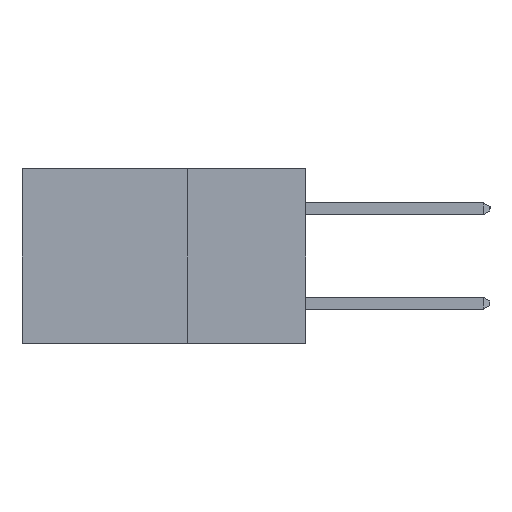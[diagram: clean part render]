
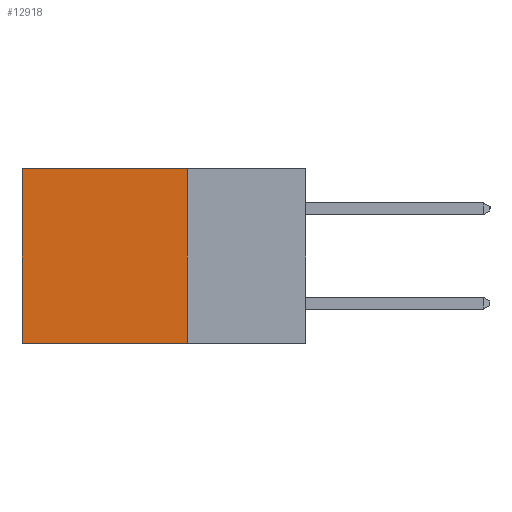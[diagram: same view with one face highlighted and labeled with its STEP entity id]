
A CAD part, left-side view. The second image highlights one B-rep face of the part: STEP entity #12918.
In plain terms, the highlighted planar face has unit normal (-1, 0, 0).
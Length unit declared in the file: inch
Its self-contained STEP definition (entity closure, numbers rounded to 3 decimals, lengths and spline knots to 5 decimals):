
#1525 = ORIENTED_EDGE ( 'NONE', *, *, #2690, .T. ) ;
#2541 = LINE ( 'NONE', #11720, #13018 ) ;
#2690 = EDGE_CURVE ( 'NONE', #2860, #10232, #7359, .T. ) ;
#2860 = VERTEX_POINT ( 'NONE', #13825 ) ;
#4169 = CARTESIAN_POINT ( 'NONE',  ( 0.2615, 0.6, -0.37 ) ) ;
#4185 = CARTESIAN_POINT ( 'NONE',  ( 0.2615, 0.25, 0. ) ) ;
#5873 = EDGE_CURVE ( 'NONE', #12660, #2860, #21415, .T. ) ;
#7359 = LINE ( 'NONE', #4169, #22644 ) ;
#7430 = CARTESIAN_POINT ( 'NONE',  ( 0.2615, 0.6, -0.37 ) ) ;
#7986 = CARTESIAN_POINT ( 'NONE',  ( 0.2615, 0.25, -0.37 ) ) ;
#9679 = DIRECTION ( 'NONE',  ( 0., 0., -1. ) ) ;
#10232 = VERTEX_POINT ( 'NONE', #7430 ) ;
#10537 = EDGE_CURVE ( 'NONE', #14693, #10232, #18271, .T. ) ;
#10885 = DIRECTION ( 'NONE',  ( 1., 0., 0. ) ) ;
#11645 = DIRECTION ( 'NONE',  ( 0., 1., 0. ) ) ;
#11720 = CARTESIAN_POINT ( 'NONE',  ( 0.2615, 0.25, -0.37 ) ) ;
#12596 = PLANE ( 'NONE',  #15592 ) ;
#12657 = ORIENTED_EDGE ( 'NONE', *, *, #5873, .T. ) ;
#12660 = VERTEX_POINT ( 'NONE', #24135 ) ;
#12918 = ADVANCED_FACE ( 'NONE', ( #16157 ), #12596, .F. ) ;
#13018 = VECTOR ( 'NONE', #19169, 39.37008 ) ;
#13825 = CARTESIAN_POINT ( 'NONE',  ( 0.2615, 0.6, 0. ) ) ;
#14242 = ORIENTED_EDGE ( 'NONE', *, *, #21147, .F. ) ;
#14329 = ORIENTED_EDGE ( 'NONE', *, *, #10537, .F. ) ;
#14563 = DIRECTION ( 'NONE',  ( 0., 0., -1. ) ) ;
#14693 = VERTEX_POINT ( 'NONE', #7986 ) ;
#15592 = AXIS2_PLACEMENT_3D ( 'NONE', #21778, #10885, #14563 ) ;
#16157 = FACE_OUTER_BOUND ( 'NONE', #22348, .T. ) ;
#16574 = DIRECTION ( 'NONE',  ( 0., 1., 0. ) ) ;
#18271 = LINE ( 'NONE', #18407, #18646 ) ;
#18407 = CARTESIAN_POINT ( 'NONE',  ( 0.2615, 0.25, -0.37 ) ) ;
#18646 = VECTOR ( 'NONE', #16574, 39.37008 ) ;
#19169 = DIRECTION ( 'NONE',  ( 0., 0., -1. ) ) ;
#21147 = EDGE_CURVE ( 'NONE', #12660, #14693, #2541, .T. ) ;
#21415 = LINE ( 'NONE', #4185, #22740 ) ;
#21778 = CARTESIAN_POINT ( 'NONE',  ( 0.2615, 0.25, -0.37 ) ) ;
#22348 = EDGE_LOOP ( 'NONE', ( #1525, #14329, #14242, #12657 ) ) ;
#22644 = VECTOR ( 'NONE', #9679, 39.37008 ) ;
#22740 = VECTOR ( 'NONE', #11645, 39.37008 ) ;
#24135 = CARTESIAN_POINT ( 'NONE',  ( 0.2615, 0.25, 0. ) ) ;
